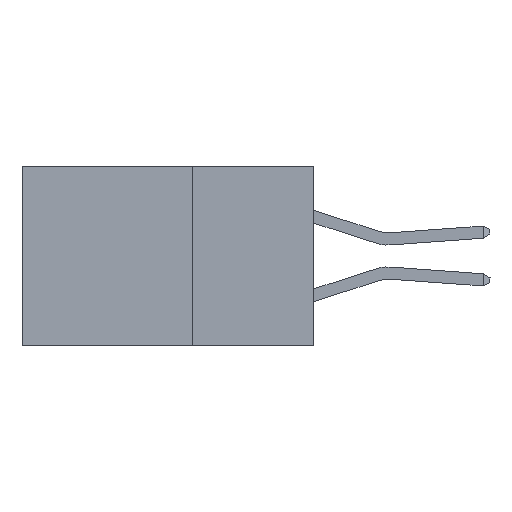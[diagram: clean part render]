
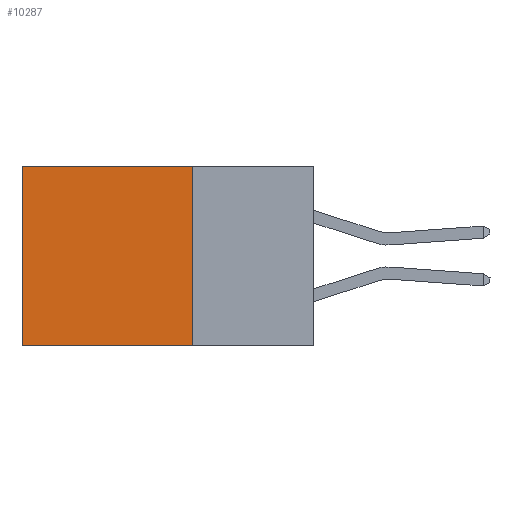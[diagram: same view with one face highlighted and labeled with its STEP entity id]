
A CAD part, left-side view. The second image highlights one B-rep face of the part: STEP entity #10287.
In plain terms, the highlighted planar face has unit normal (-1, 0, 0).
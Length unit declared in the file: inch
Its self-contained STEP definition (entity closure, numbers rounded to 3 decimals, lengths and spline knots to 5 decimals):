
#925 = DIRECTION ( 'NONE',  ( 0., 0., -1. ) ) ;
#1440 = AXIS2_PLACEMENT_3D ( 'NONE', #14974, #8329, #8135 ) ;
#1792 = CARTESIAN_POINT ( 'NONE',  ( 0.2875, 0.25, 0. ) ) ;
#1916 = EDGE_CURVE ( 'NONE', #23055, #24075, #20514, .T. ) ;
#2250 = EDGE_CURVE ( 'NONE', #12059, #12051, #12186, .T. ) ;
#3437 = VECTOR ( 'NONE', #5281, 39.37008 ) ;
#4410 = VECTOR ( 'NONE', #27965, 39.37008 ) ;
#5281 = DIRECTION ( 'NONE',  ( 0., 1., 0. ) ) ;
#7836 = LINE ( 'NONE', #8169, #4410 ) ;
#8135 = DIRECTION ( 'NONE',  ( 0., 0., -1. ) ) ;
#8169 = CARTESIAN_POINT ( 'NONE',  ( 0.2875, 0.25, 0. ) ) ;
#8329 = DIRECTION ( 'NONE',  ( 1., 0., 0. ) ) ;
#9652 = EDGE_CURVE ( 'NONE', #12059, #23055, #7836, .T. ) ;
#10202 = FACE_OUTER_BOUND ( 'NONE', #15562, .T. ) ;
#10287 = ADVANCED_FACE ( 'NONE', ( #10202 ), #19506, .F. ) ;
#10590 = CARTESIAN_POINT ( 'NONE',  ( 0.2875, 0.6, -0.37 ) ) ;
#11420 = ORIENTED_EDGE ( 'NONE', *, *, #2250, .F. ) ;
#11918 = CARTESIAN_POINT ( 'NONE',  ( 0.2875, 0.25, 0. ) ) ;
#12051 = VERTEX_POINT ( 'NONE', #25178 ) ;
#12059 = VERTEX_POINT ( 'NONE', #11918 ) ;
#12186 = LINE ( 'NONE', #1792, #17387 ) ;
#14913 = ORIENTED_EDGE ( 'NONE', *, *, #25602, .F. ) ;
#14974 = CARTESIAN_POINT ( 'NONE',  ( 0.2875, 0.25, 0. ) ) ;
#15562 = EDGE_LOOP ( 'NONE', ( #19729, #14913, #11420, #23209 ) ) ;
#16722 = VECTOR ( 'NONE', #925, 39.37008 ) ;
#17387 = VECTOR ( 'NONE', #23943, 39.37008 ) ;
#17802 = CARTESIAN_POINT ( 'NONE',  ( 0.2875, 0.6, 0. ) ) ;
#17981 = CARTESIAN_POINT ( 'NONE',  ( 0.2875, 0.25, -0.37 ) ) ;
#19506 = PLANE ( 'NONE',  #1440 ) ;
#19729 = ORIENTED_EDGE ( 'NONE', *, *, #1916, .T. ) ;
#20514 = LINE ( 'NONE', #22793, #16722 ) ;
#22793 = CARTESIAN_POINT ( 'NONE',  ( 0.2875, 0.6, 0. ) ) ;
#23055 = VERTEX_POINT ( 'NONE', #17802 ) ;
#23209 = ORIENTED_EDGE ( 'NONE', *, *, #9652, .T. ) ;
#23761 = LINE ( 'NONE', #17981, #3437 ) ;
#23943 = DIRECTION ( 'NONE',  ( 0., 0., -1. ) ) ;
#24075 = VERTEX_POINT ( 'NONE', #10590 ) ;
#25178 = CARTESIAN_POINT ( 'NONE',  ( 0.2875, 0.25, -0.37 ) ) ;
#25602 = EDGE_CURVE ( 'NONE', #12051, #24075, #23761, .T. ) ;
#27965 = DIRECTION ( 'NONE',  ( 0., 1., 0. ) ) ;
